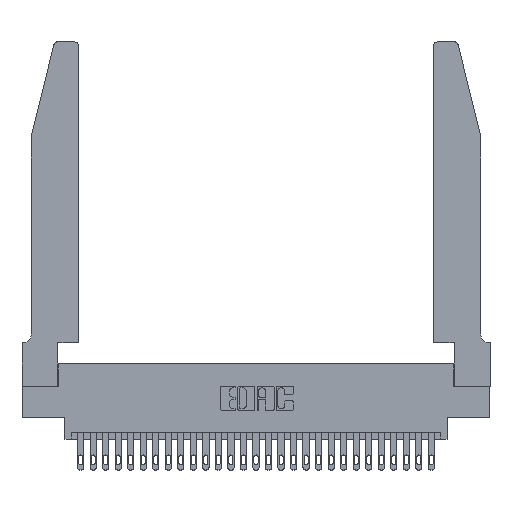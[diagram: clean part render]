
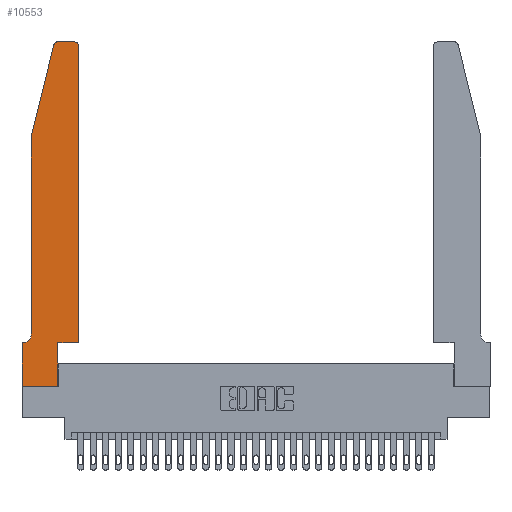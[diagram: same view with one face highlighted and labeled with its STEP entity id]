
A CAD part, top view. The second image highlights one B-rep face of the part: STEP entity #10553.
In plain terms, the highlighted planar face has unit normal (0, 0, 1).
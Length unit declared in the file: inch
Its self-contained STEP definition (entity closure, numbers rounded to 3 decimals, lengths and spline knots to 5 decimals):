
#48 = AXIS2_PLACEMENT_3D ( 'NONE', #6156, #14933, #28830 ) ;
#485 = EDGE_CURVE ( 'NONE', #25951, #15460, #10053, .T. ) ;
#743 = ORIENTED_EDGE ( 'NONE', *, *, #485, .T. ) ;
#1195 = VERTEX_POINT ( 'NONE', #4395 ) ;
#1250 = LINE ( 'NONE', #26198, #8024 ) ;
#1458 = EDGE_LOOP ( 'NONE', ( #5910, #18987, #743, #10776, #8890, #25110, #12983, #9009, #23579, #26678, #15402, #14208 ) ) ;
#1609 = CARTESIAN_POINT ( 'NONE',  ( 0.25487, 2.72718, 0.37 ) ) ;
#1719 = AXIS2_PLACEMENT_3D ( 'NONE', #2376, #13458, #11386 ) ;
#1836 = CARTESIAN_POINT ( 'NONE',  ( 0.2865, 0.35, 0.37 ) ) ;
#1911 = VECTOR ( 'NONE', #7604, 39.37008 ) ;
#2177 = LINE ( 'NONE', #1836, #22078 ) ;
#2376 = CARTESIAN_POINT ( 'NONE',  ( 0.0055, 0.42, 0.37 ) ) ;
#3165 = VECTOR ( 'NONE', #5223, 39.37008 ) ;
#3284 = EDGE_CURVE ( 'NONE', #6619, #5207, #23964, .T. ) ;
#3537 = DIRECTION ( 'NONE',  ( 0., -1., 0. ) ) ;
#3628 = DIRECTION ( 'NONE',  ( 0., 0., 1. ) ) ;
#4377 = DIRECTION ( 'NONE',  ( 1., 0., 0. ) ) ;
#4395 = CARTESIAN_POINT ( 'NONE',  ( 0., 0., 0.37 ) ) ;
#5207 = VERTEX_POINT ( 'NONE', #6356 ) ;
#5223 = DIRECTION ( 'NONE',  ( 1., 0., 0. ) ) ;
#5910 = ORIENTED_EDGE ( 'NONE', *, *, #7047, .T. ) ;
#5950 = LINE ( 'NONE', #26741, #14060 ) ;
#6059 = CARTESIAN_POINT ( 'NONE',  ( 0.0055, 0.35, 0.37 ) ) ;
#6156 = CARTESIAN_POINT ( 'NONE',  ( 0.4205, 2.72, 0.37 ) ) ;
#6356 = CARTESIAN_POINT ( 'NONE',  ( 0.4205, 2.75, 0.37 ) ) ;
#6516 = CARTESIAN_POINT ( 'NONE',  ( 0., 0.35, 0.37 ) ) ;
#6619 = VERTEX_POINT ( 'NONE', #9608 ) ;
#7047 = EDGE_CURVE ( 'NONE', #5207, #13206, #13079, .T. ) ;
#7054 = CARTESIAN_POINT ( 'NONE',  ( 0.4505, 0.35, 0.37 ) ) ;
#7179 = DIRECTION ( 'NONE',  ( -0.239, -0.971, 0. ) ) ;
#7604 = DIRECTION ( 'NONE',  ( 0., 1., 0. ) ) ;
#8024 = VECTOR ( 'NONE', #3537, 39.37008 ) ;
#8127 = EDGE_CURVE ( 'NONE', #13974, #22919, #5950, .T. ) ;
#8223 = CARTESIAN_POINT ( 'NONE',  ( 0.284, 2.72, 0.37 ) ) ;
#8510 = EDGE_CURVE ( 'NONE', #15460, #20528, #11923, .T. ) ;
#8749 = CARTESIAN_POINT ( 'NONE',  ( 0., 0.35, 0.37 ) ) ;
#8807 = DIRECTION ( 'NONE',  ( 0., 1., 0. ) ) ;
#8863 = VECTOR ( 'NONE', #11348, 39.37008 ) ;
#8890 = ORIENTED_EDGE ( 'NONE', *, *, #17753, .T. ) ;
#9009 = ORIENTED_EDGE ( 'NONE', *, *, #11848, .T. ) ;
#9092 = VERTEX_POINT ( 'NONE', #14308 ) ;
#9475 = EDGE_CURVE ( 'NONE', #9092, #13974, #2177, .T. ) ;
#9484 = VECTOR ( 'NONE', #10122, 39.37008 ) ;
#9608 = CARTESIAN_POINT ( 'NONE',  ( 0.4505, 2.72, 0.37 ) ) ;
#10053 = LINE ( 'NONE', #25170, #27409 ) ;
#10122 = DIRECTION ( 'NONE',  ( -1., 0., 0. ) ) ;
#10553 = ADVANCED_FACE ( 'NONE', ( #25536 ), #20037, .T. ) ;
#10776 = ORIENTED_EDGE ( 'NONE', *, *, #8510, .T. ) ;
#10892 = DIRECTION ( 'NONE',  ( 1., 0., 0. ) ) ;
#11348 = DIRECTION ( 'NONE',  ( -1., 0., 0. ) ) ;
#11386 = DIRECTION ( 'NONE',  ( -1., 0., 0. ) ) ;
#11544 = CARTESIAN_POINT ( 'NONE',  ( 0.2605, 2.75, 0.37 ) ) ;
#11848 = EDGE_CURVE ( 'NONE', #1195, #9092, #22338, .T. ) ;
#11923 = LINE ( 'NONE', #16559, #17628 ) ;
#12373 = VERTEX_POINT ( 'NONE', #6516 ) ;
#12461 = CARTESIAN_POINT ( 'NONE',  ( 0.0755, 2., 0.37 ) ) ;
#12983 = ORIENTED_EDGE ( 'NONE', *, *, #13959, .T. ) ;
#13079 = LINE ( 'NONE', #11544, #8863 ) ;
#13206 = VERTEX_POINT ( 'NONE', #16761 ) ;
#13458 = DIRECTION ( 'NONE',  ( 0., 0., -1. ) ) ;
#13959 = EDGE_CURVE ( 'NONE', #12373, #1195, #1250, .T. ) ;
#13974 = VERTEX_POINT ( 'NONE', #21799 ) ;
#14060 = VECTOR ( 'NONE', #4377, 39.37008 ) ;
#14208 = ORIENTED_EDGE ( 'NONE', *, *, #3284, .T. ) ;
#14308 = CARTESIAN_POINT ( 'NONE',  ( 0.2865, 0., 0.37 ) ) ;
#14933 = DIRECTION ( 'NONE',  ( 0., 0., 1. ) ) ;
#15389 = AXIS2_PLACEMENT_3D ( 'NONE', #8223, #3628, #24046 ) ;
#15402 = ORIENTED_EDGE ( 'NONE', *, *, #25821, .T. ) ;
#15460 = VERTEX_POINT ( 'NONE', #12461 ) ;
#15528 = VERTEX_POINT ( 'NONE', #6059 ) ;
#16559 = CARTESIAN_POINT ( 'NONE',  ( 0.0755, 2., 0.37 ) ) ;
#16691 = CARTESIAN_POINT ( 'NONE',  ( 0.4505, 0.35, 0.37 ) ) ;
#16761 = CARTESIAN_POINT ( 'NONE',  ( 0.284, 2.75, 0.37 ) ) ;
#16968 = CARTESIAN_POINT ( 'NONE',  ( 0.0755, 0.35, 0.37 ) ) ;
#17628 = VECTOR ( 'NONE', #21229, 39.37008 ) ;
#17753 = EDGE_CURVE ( 'NONE', #20528, #15528, #26239, .T. ) ;
#18766 = EDGE_CURVE ( 'NONE', #13206, #25951, #27594, .T. ) ;
#18987 = ORIENTED_EDGE ( 'NONE', *, *, #18766, .T. ) ;
#19065 = LINE ( 'NONE', #16968, #9484 ) ;
#20037 = PLANE ( 'NONE',  #25741 ) ;
#20400 = EDGE_CURVE ( 'NONE', #15528, #12373, #19065, .T. ) ;
#20528 = VERTEX_POINT ( 'NONE', #28849 ) ;
#21229 = DIRECTION ( 'NONE',  ( 0., -1., 0. ) ) ;
#21799 = CARTESIAN_POINT ( 'NONE',  ( 0.2865, 0.35, 0.37 ) ) ;
#22078 = VECTOR ( 'NONE', #8807, 39.37008 ) ;
#22338 = LINE ( 'NONE', #28005, #3165 ) ;
#22555 = LINE ( 'NONE', #16691, #1911 ) ;
#22919 = VERTEX_POINT ( 'NONE', #7054 ) ;
#23579 = ORIENTED_EDGE ( 'NONE', *, *, #9475, .T. ) ;
#23964 = CIRCLE ( 'NONE', #48, 0.03 ) ;
#24046 = DIRECTION ( 'NONE',  ( 1., 0., 0. ) ) ;
#25110 = ORIENTED_EDGE ( 'NONE', *, *, #20400, .T. ) ;
#25170 = CARTESIAN_POINT ( 'NONE',  ( 0.0755, 2., 0.37 ) ) ;
#25536 = FACE_OUTER_BOUND ( 'NONE', #1458, .T. ) ;
#25741 = AXIS2_PLACEMENT_3D ( 'NONE', #8749, #26818, #10892 ) ;
#25821 = EDGE_CURVE ( 'NONE', #22919, #6619, #22555, .T. ) ;
#25951 = VERTEX_POINT ( 'NONE', #1609 ) ;
#26198 = CARTESIAN_POINT ( 'NONE',  ( 0., 0., 0.37 ) ) ;
#26239 = CIRCLE ( 'NONE', #1719, 0.07 ) ;
#26678 = ORIENTED_EDGE ( 'NONE', *, *, #8127, .T. ) ;
#26741 = CARTESIAN_POINT ( 'NONE',  ( 0.4505, 0.35, 0.37 ) ) ;
#26818 = DIRECTION ( 'NONE',  ( 0., 0., 1. ) ) ;
#27409 = VECTOR ( 'NONE', #7179, 39.37008 ) ;
#27594 = CIRCLE ( 'NONE', #15389, 0.03 ) ;
#28005 = CARTESIAN_POINT ( 'NONE',  ( 0., 0., 0.37 ) ) ;
#28830 = DIRECTION ( 'NONE',  ( 1., 0., 0. ) ) ;
#28849 = CARTESIAN_POINT ( 'NONE',  ( 0.0755, 0.42, 0.37 ) ) ;
